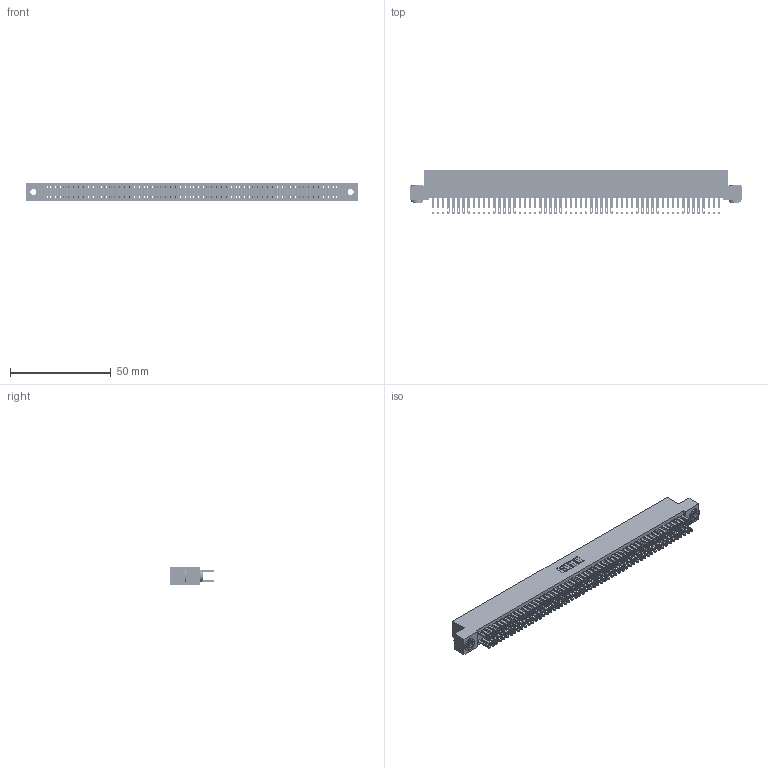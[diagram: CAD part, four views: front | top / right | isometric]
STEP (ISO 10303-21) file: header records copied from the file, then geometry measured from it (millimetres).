
FILE_DESCRIPTION (( 'STEP AP203' ), '1' );
FILE_NAME ('892-114-500-203.STEP', '2020-09-21T22:07:08', ( '' ), ( '' ), 'SwSTEP 2.0', 'SolidWorks 2020', '' );
FILE_SCHEMA (( 'CONFIG_CONTROL_DESIGN' ));
Length unit declared in the file: inch
Products named in the file (4): 345-292-001_345-293-100; 342-250-002_345-250-002-102; 892-114-500-203; 842 Part_.156 TH
Assembly tree (117 placements, depth 2):
  892-114-500-203
    842 Part_.156 TH
    345-292-001_345-293-100  x114
    342-250-002_345-250-002-102  x2
Bounding box: 165.1 x 21.85 x 9.4 mm (x, y, z)
Volume: 15276.4 mm3; surface area: 26541.3 mm2
Topology: 117 solids, 117 shells, 5620 faces, 17133 edges, 11418 vertices
Faces by surface type: plane 3496, cylinder 2116, cone 8
Entity records: 35178 total; most frequent: CARTESIAN_POINT 5785, ORIENTED_EDGE 5714, DIRECTION 4951, EDGE_CURVE 2857, VECTOR 2701, LINE 2701, VERTEX_POINT 1902, AXIS2_PLACEMENT_3D 1125
